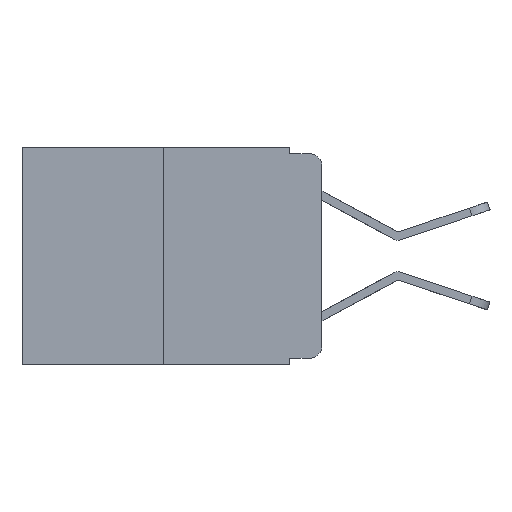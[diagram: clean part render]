
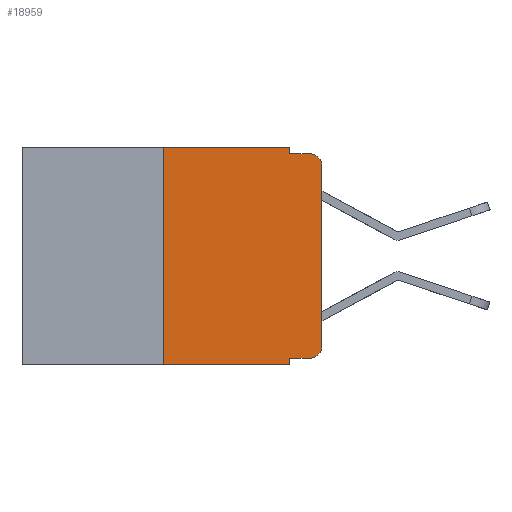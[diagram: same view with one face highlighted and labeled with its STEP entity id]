
A CAD part, left-side view. The second image highlights one B-rep face of the part: STEP entity #18959.
In plain terms, the highlighted planar face has unit normal (-1, 0, 0).
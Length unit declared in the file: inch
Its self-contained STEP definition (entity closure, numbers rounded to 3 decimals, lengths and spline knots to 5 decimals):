
#26 = CARTESIAN_POINT ( 'NONE',  ( 0., 0.051, -0.343 ) ) ;
#279 = CARTESIAN_POINT ( 'NONE',  ( 0., 0.051, -0.01 ) ) ;
#349 = VERTEX_POINT ( 'NONE', #19290 ) ;
#411 = LINE ( 'NONE', #9012, #12266 ) ;
#881 = VERTEX_POINT ( 'NONE', #8437 ) ;
#1008 = VERTEX_POINT ( 'NONE', #26 ) ;
#1198 = CARTESIAN_POINT ( 'NONE',  ( 0., 0.25, 0. ) ) ;
#1409 = VECTOR ( 'NONE', #9668, 39.37008 ) ;
#1453 = CARTESIAN_POINT ( 'NONE',  ( 0., 0.473, 0. ) ) ;
#1599 = ORIENTED_EDGE ( 'NONE', *, *, #3305, .T. ) ;
#1773 = ORIENTED_EDGE ( 'NONE', *, *, #4646, .T. ) ;
#1898 = VERTEX_POINT ( 'NONE', #23067 ) ;
#2190 = VECTOR ( 'NONE', #8083, 39.37008 ) ;
#3305 = EDGE_CURVE ( 'NONE', #1898, #349, #19409, .T. ) ;
#3360 = DIRECTION ( 'NONE',  ( 0., 0., -1. ) ) ;
#3500 = VECTOR ( 'NONE', #6034, 39.37008 ) ;
#4404 = CARTESIAN_POINT ( 'NONE',  ( 0., 0.02, -0.03 ) ) ;
#4408 = DIRECTION ( 'NONE',  ( 0., -1., 0. ) ) ;
#4474 = EDGE_CURVE ( 'NONE', #4548, #9523, #17166, .T. ) ;
#4548 = VERTEX_POINT ( 'NONE', #16336 ) ;
#4646 = EDGE_CURVE ( 'NONE', #349, #21573, #13083, .T. ) ;
#5269 = CARTESIAN_POINT ( 'NONE',  ( 0., 0.051, -0.333 ) ) ;
#5553 = CARTESIAN_POINT ( 'NONE',  ( 0., 0.25, 0. ) ) ;
#6034 = DIRECTION ( 'NONE',  ( 0., -1., 0. ) ) ;
#6348 = DIRECTION ( 'NONE',  ( 0., 0., -1. ) ) ;
#6443 = CARTESIAN_POINT ( 'NONE',  ( 0., 0., 0. ) ) ;
#7167 = PLANE ( 'NONE',  #12025 ) ;
#7186 = LINE ( 'NONE', #1198, #16455 ) ;
#7542 = EDGE_CURVE ( 'NONE', #881, #22534, #7186, .T. ) ;
#8083 = DIRECTION ( 'NONE',  ( 0., 0., -1. ) ) ;
#8437 = CARTESIAN_POINT ( 'NONE',  ( 0., 0.25, -0.343 ) ) ;
#8522 = CARTESIAN_POINT ( 'NONE',  ( 0., 0., -0.03 ) ) ;
#8661 = VERTEX_POINT ( 'NONE', #5269 ) ;
#9012 = CARTESIAN_POINT ( 'NONE',  ( 0., 0.051, 0. ) ) ;
#9523 = VERTEX_POINT ( 'NONE', #279 ) ;
#9668 = DIRECTION ( 'NONE',  ( 0., -1., 0. ) ) ;
#10476 = EDGE_CURVE ( 'NONE', #8661, #1008, #411, .T. ) ;
#10487 = ORIENTED_EDGE ( 'NONE', *, *, #23214, .T. ) ;
#10774 = CARTESIAN_POINT ( 'NONE',  ( 0., 0.02, -0.313 ) ) ;
#10974 = DIRECTION ( 'NONE',  ( -1., 0., 0. ) ) ;
#10978 = DIRECTION ( 'NONE',  ( 0., 0., -1. ) ) ;
#11325 = VERTEX_POINT ( 'NONE', #18351 ) ;
#11420 = AXIS2_PLACEMENT_3D ( 'NONE', #10774, #10974, #10978 ) ;
#12025 = AXIS2_PLACEMENT_3D ( 'NONE', #1453, #14607, #3360 ) ;
#12266 = VECTOR ( 'NONE', #21854, 39.37008 ) ;
#13083 = LINE ( 'NONE', #6443, #17442 ) ;
#13144 = CIRCLE ( 'NONE', #17612, 0.02 ) ;
#13453 = LINE ( 'NONE', #15616, #18362 ) ;
#14067 = LINE ( 'NONE', #17191, #3500 ) ;
#14138 = ORIENTED_EDGE ( 'NONE', *, *, #20212, .T. ) ;
#14436 = EDGE_CURVE ( 'NONE', #22534, #4548, #19556, .T. ) ;
#14515 = EDGE_CURVE ( 'NONE', #881, #1008, #14067, .T. ) ;
#14607 = DIRECTION ( 'NONE',  ( 1., 0., 0. ) ) ;
#15616 = CARTESIAN_POINT ( 'NONE',  ( 0., 0.051, -0.333 ) ) ;
#16336 = CARTESIAN_POINT ( 'NONE',  ( 0., 0.051, 0. ) ) ;
#16455 = VECTOR ( 'NONE', #19765, 39.37008 ) ;
#16665 = DIRECTION ( 'NONE',  ( 0., 0., 1. ) ) ;
#17166 = LINE ( 'NONE', #22253, #2190 ) ;
#17191 = CARTESIAN_POINT ( 'NONE',  ( 0., 0.473, -0.343 ) ) ;
#17442 = VECTOR ( 'NONE', #16665, 39.37008 ) ;
#17480 = DIRECTION ( 'NONE',  ( -1., 0., 0. ) ) ;
#17612 = AXIS2_PLACEMENT_3D ( 'NONE', #4404, #17480, #6348 ) ;
#18351 = CARTESIAN_POINT ( 'NONE',  ( 0., 0.02, -0.01 ) ) ;
#18362 = VECTOR ( 'NONE', #4408, 39.37008 ) ;
#18551 = ORIENTED_EDGE ( 'NONE', *, *, #10476, .F. ) ;
#18757 = CARTESIAN_POINT ( 'NONE',  ( 0., 0.051, -0.01 ) ) ;
#18867 = CARTESIAN_POINT ( 'NONE',  ( 0., 0.473, 0. ) ) ;
#18959 = ADVANCED_FACE ( 'NONE', ( #21802 ), #7167, .F. ) ;
#19290 = CARTESIAN_POINT ( 'NONE',  ( 0., 0., -0.313 ) ) ;
#19409 = CIRCLE ( 'NONE', #11420, 0.02 ) ;
#19556 = LINE ( 'NONE', #18867, #1409 ) ;
#19683 = ORIENTED_EDGE ( 'NONE', *, *, #14436, .F. ) ;
#19765 = DIRECTION ( 'NONE',  ( 0., 0., 1. ) ) ;
#20212 = EDGE_CURVE ( 'NONE', #21573, #11325, #13144, .T. ) ;
#21054 = ORIENTED_EDGE ( 'NONE', *, *, #4474, .F. ) ;
#21214 = VECTOR ( 'NONE', #22479, 39.37008 ) ;
#21573 = VERTEX_POINT ( 'NONE', #8522 ) ;
#21776 = LINE ( 'NONE', #18757, #21214 ) ;
#21802 = FACE_OUTER_BOUND ( 'NONE', #22953, .T. ) ;
#21854 = DIRECTION ( 'NONE',  ( 0., 0., -1. ) ) ;
#21878 = ORIENTED_EDGE ( 'NONE', *, *, #23083, .F. ) ;
#21903 = ORIENTED_EDGE ( 'NONE', *, *, #14515, .T. ) ;
#22253 = CARTESIAN_POINT ( 'NONE',  ( 0., 0.051, 0. ) ) ;
#22479 = DIRECTION ( 'NONE',  ( 0., -1., 0. ) ) ;
#22534 = VERTEX_POINT ( 'NONE', #5553 ) ;
#22737 = ORIENTED_EDGE ( 'NONE', *, *, #7542, .F. ) ;
#22953 = EDGE_LOOP ( 'NONE', ( #1773, #14138, #21878, #21054, #19683, #22737, #21903, #18551, #10487, #1599 ) ) ;
#23067 = CARTESIAN_POINT ( 'NONE',  ( 0., 0.02, -0.333 ) ) ;
#23083 = EDGE_CURVE ( 'NONE', #9523, #11325, #21776, .T. ) ;
#23214 = EDGE_CURVE ( 'NONE', #8661, #1898, #13453, .T. ) ;
